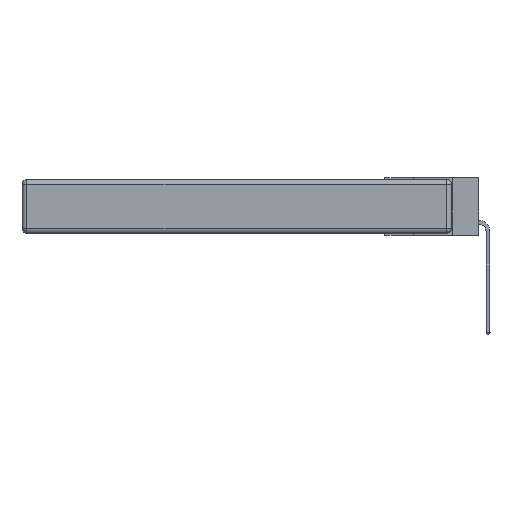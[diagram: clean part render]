
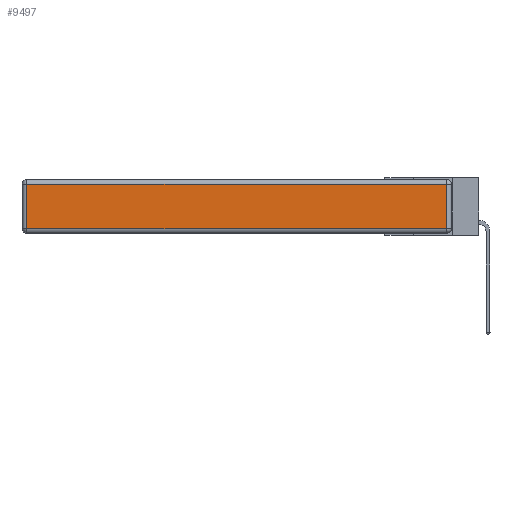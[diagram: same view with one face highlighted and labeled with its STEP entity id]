
A CAD part, left-side view. The second image highlights one B-rep face of the part: STEP entity #9497.
In plain terms, the highlighted planar face has unit normal (-1, 0, 0).
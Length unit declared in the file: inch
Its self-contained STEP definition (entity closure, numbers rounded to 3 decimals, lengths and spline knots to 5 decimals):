
#270 = VECTOR ( 'NONE', #9362, 39.37008 ) ;
#676 = CARTESIAN_POINT ( 'NONE',  ( 0., 2.75, -0.03 ) ) ;
#705 = AXIS2_PLACEMENT_3D ( 'NONE', #8382, #908, #7476 ) ;
#908 = DIRECTION ( 'NONE',  ( -1., 0., 0. ) ) ;
#1031 = DIRECTION ( 'NONE',  ( 0., 0., 1. ) ) ;
#1349 = DIRECTION ( 'NONE',  ( 0., 0., -1. ) ) ;
#1982 = EDGE_CURVE ( 'NONE', #3222, #9332, #6529, .T. ) ;
#2601 = ORIENTED_EDGE ( 'NONE', *, *, #1982, .T. ) ;
#3011 = FACE_OUTER_BOUND ( 'NONE', #9184, .T. ) ;
#3222 = VERTEX_POINT ( 'NONE', #9301 ) ;
#3570 = EDGE_CURVE ( 'NONE', #4590, #3222, #6748, .T. ) ;
#3811 = LINE ( 'NONE', #5979, #4821 ) ;
#4465 = CARTESIAN_POINT ( 'NONE',  ( 0., 0.03, -0.03 ) ) ;
#4590 = VERTEX_POINT ( 'NONE', #7765 ) ;
#4757 = ORIENTED_EDGE ( 'NONE', *, *, #8896, .T. ) ;
#4821 = VECTOR ( 'NONE', #1349, 39.37008 ) ;
#5865 = CARTESIAN_POINT ( 'NONE',  ( 0., 2.72, -0.03 ) ) ;
#5979 = CARTESIAN_POINT ( 'NONE',  ( 0., 2.72, -0.343 ) ) ;
#6027 = DIRECTION ( 'NONE',  ( 0., -1., 0. ) ) ;
#6511 = EDGE_CURVE ( 'NONE', #11909, #4590, #3811, .T. ) ;
#6529 = LINE ( 'NONE', #9480, #12108 ) ;
#6748 = LINE ( 'NONE', #7953, #9231 ) ;
#7427 = PLANE ( 'NONE',  #705 ) ;
#7476 = DIRECTION ( 'NONE',  ( 0., 0., 1. ) ) ;
#7765 = CARTESIAN_POINT ( 'NONE',  ( 0., 2.72, -0.313 ) ) ;
#7953 = CARTESIAN_POINT ( 'NONE',  ( 0., 0., -0.313 ) ) ;
#8127 = LINE ( 'NONE', #676, #270 ) ;
#8382 = CARTESIAN_POINT ( 'NONE',  ( 0., 0., -0.343 ) ) ;
#8502 = ORIENTED_EDGE ( 'NONE', *, *, #6511, .T. ) ;
#8896 = EDGE_CURVE ( 'NONE', #9332, #11909, #8127, .T. ) ;
#9184 = EDGE_LOOP ( 'NONE', ( #12027, #2601, #4757, #8502 ) ) ;
#9231 = VECTOR ( 'NONE', #6027, 39.37008 ) ;
#9301 = CARTESIAN_POINT ( 'NONE',  ( 0., 0.03, -0.313 ) ) ;
#9332 = VERTEX_POINT ( 'NONE', #4465 ) ;
#9362 = DIRECTION ( 'NONE',  ( 0., 1., 0. ) ) ;
#9480 = CARTESIAN_POINT ( 'NONE',  ( 0., 0.03, -0.343 ) ) ;
#9497 = ADVANCED_FACE ( 'NONE', ( #3011 ), #7427, .T. ) ;
#11909 = VERTEX_POINT ( 'NONE', #5865 ) ;
#12027 = ORIENTED_EDGE ( 'NONE', *, *, #3570, .T. ) ;
#12108 = VECTOR ( 'NONE', #1031, 39.37008 ) ;
